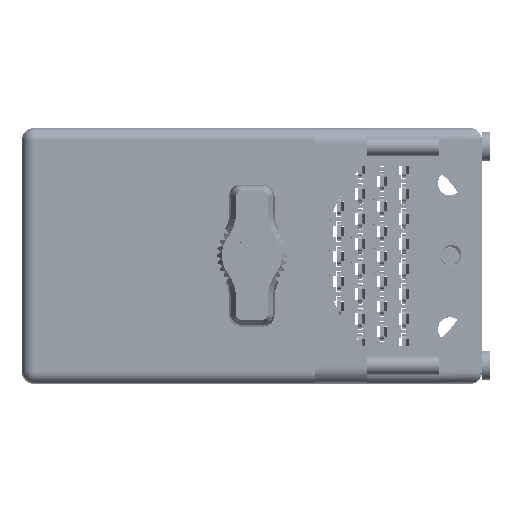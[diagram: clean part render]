
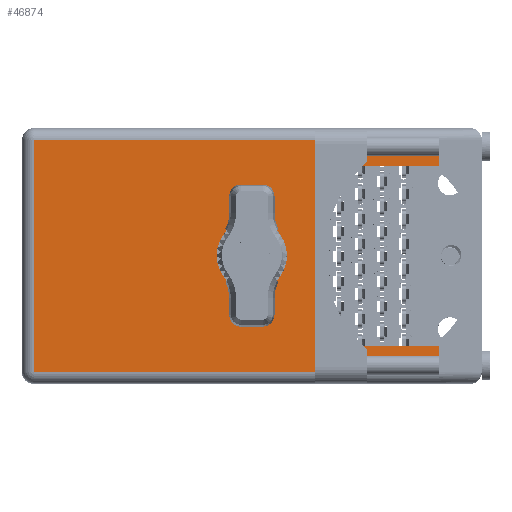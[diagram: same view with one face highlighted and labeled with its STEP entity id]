
A CAD part, top view. The second image highlights one B-rep face of the part: STEP entity #46874.
In plain terms, the highlighted face is planar.
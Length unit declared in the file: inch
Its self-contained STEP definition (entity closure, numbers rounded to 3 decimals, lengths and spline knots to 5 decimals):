
#1125 = AXIS2_PLACEMENT_3D ( 'NONE', #104734, #112836, #76635 ) ;
#4135 = VECTOR ( 'NONE', #70234, 39.37008 ) ;
#5523 = LINE ( 'NONE', #11830, #114775 ) ;
#6283 = VERTEX_POINT ( 'NONE', #26137 ) ;
#6298 = ORIENTED_EDGE ( 'NONE', *, *, #83334, .T. ) ;
#6409 = CARTESIAN_POINT ( 'NONE',  ( 0., 2.03, -1.46 ) ) ;
#7267 = EDGE_LOOP ( 'NONE', ( #102553, #46336, #51465, #106313, #6298, #98433, #116353, #37345 ) ) ;
#8203 = FACE_OUTER_BOUND ( 'NONE', #7267, .T. ) ;
#11830 = CARTESIAN_POINT ( 'NONE',  ( 2.499, 2.03, -1.53 ) ) ;
#12040 = VERTEX_POINT ( 'NONE', #65468 ) ;
#12286 = DIRECTION ( 'NONE',  ( 0., 0., 1. ) ) ;
#13913 = DIRECTION ( 'NONE',  ( 1., 0., 0. ) ) ;
#14869 = AXIS2_PLACEMENT_3D ( 'NONE', #26326, #91698, #35179 ) ;
#18072 = EDGE_CURVE ( 'NONE', #61223, #6283, #25681, .T. ) ;
#21875 = LINE ( 'NONE', #77321, #57810 ) ;
#22749 = CARTESIAN_POINT ( 'NONE',  ( 1.785, 2.03, -1.305 ) ) ;
#23350 = CARTESIAN_POINT ( 'NONE',  ( 2.499, 2.03, -0.07 ) ) ;
#23703 = EDGE_CURVE ( 'NONE', #98902, #97564, #72980, .T. ) ;
#24922 = CARTESIAN_POINT ( 'NONE',  ( 2.499, 2.03, -0.225 ) ) ;
#25681 = LINE ( 'NONE', #108618, #110474 ) ;
#26137 = CARTESIAN_POINT ( 'NONE',  ( 0.07, 2.03, -0.07 ) ) ;
#26326 = CARTESIAN_POINT ( 'NONE',  ( 1.3775, 2.03, -0.765 ) ) ;
#28358 = ORIENTED_EDGE ( 'NONE', *, *, #86660, .F. ) ;
#30281 = CARTESIAN_POINT ( 'NONE',  ( 0., 2.03, -1.53 ) ) ;
#33749 = VERTEX_POINT ( 'NONE', #23350 ) ;
#34765 = EDGE_CURVE ( 'NONE', #115130, #12040, #5523, .T. ) ;
#35179 = DIRECTION ( 'NONE',  ( 0., 0., 1. ) ) ;
#35689 = LINE ( 'NONE', #69709, #47110 ) ;
#36086 = CARTESIAN_POINT ( 'NONE',  ( 1.3775, 2.03, -0.595 ) ) ;
#37345 = ORIENTED_EDGE ( 'NONE', *, *, #74358, .T. ) ;
#39644 = LINE ( 'NONE', #112432, #76914 ) ;
#39777 = VERTEX_POINT ( 'NONE', #24922 ) ;
#40352 = EDGE_CURVE ( 'NONE', #39777, #45033, #72244, .T. ) ;
#44731 = VERTEX_POINT ( 'NONE', #115864 ) ;
#45033 = VERTEX_POINT ( 'NONE', #94032 ) ;
#45855 = CIRCLE ( 'NONE', #1125, 0.17 ) ;
#46336 = ORIENTED_EDGE ( 'NONE', *, *, #48049, .T. ) ;
#46874 = ADVANCED_FACE ( 'NONE', ( #8203, #78607 ), #112604, .T. ) ;
#47110 = VECTOR ( 'NONE', #13913, 39.37008 ) ;
#48049 = EDGE_CURVE ( 'NONE', #6283, #33749, #39644, .T. ) ;
#49208 = VECTOR ( 'NONE', #86919, 39.37008 ) ;
#51465 = ORIENTED_EDGE ( 'NONE', *, *, #97383, .F. ) ;
#52544 = CARTESIAN_POINT ( 'NONE',  ( 0.07, 2.03, -1.46 ) ) ;
#53623 = VECTOR ( 'NONE', #109043, 39.37008 ) ;
#57429 = DIRECTION ( 'NONE',  ( 1., 0., 0. ) ) ;
#57810 = VECTOR ( 'NONE', #12286, 39.37008 ) ;
#61223 = VERTEX_POINT ( 'NONE', #52544 ) ;
#65468 = CARTESIAN_POINT ( 'NONE',  ( 2.499, 2.03, -1.305 ) ) ;
#65656 = DIRECTION ( 'NONE',  ( 0., 0., 1. ) ) ;
#69709 = CARTESIAN_POINT ( 'NONE',  ( 2.499, 2.03, -1.305 ) ) ;
#70234 = DIRECTION ( 'NONE',  ( -1., 0., 0. ) ) ;
#72244 = LINE ( 'NONE', #107843, #53623 ) ;
#72980 = CIRCLE ( 'NONE', #14869, 0.17 ) ;
#74358 = EDGE_CURVE ( 'NONE', #115130, #61223, #111857, .T. ) ;
#74712 = EDGE_CURVE ( 'NONE', #44731, #12040, #35689, .T. ) ;
#76635 = DIRECTION ( 'NONE',  ( 0., 0., 1. ) ) ;
#76914 = VECTOR ( 'NONE', #57429, 39.37008 ) ;
#77321 = CARTESIAN_POINT ( 'NONE',  ( 2.499, 2.03, -1.53 ) ) ;
#78607 = FACE_BOUND ( 'NONE', #107904, .T. ) ;
#78667 = CARTESIAN_POINT ( 'NONE',  ( 2.499, 2.03, -1.46 ) ) ;
#83334 = EDGE_CURVE ( 'NONE', #45033, #44731, #106625, .T. ) ;
#84444 = DIRECTION ( 'NONE',  ( 0., 0., 1. ) ) ;
#86660 = EDGE_CURVE ( 'NONE', #97564, #98902, #45855, .T. ) ;
#86919 = DIRECTION ( 'NONE',  ( 0., 0., -1. ) ) ;
#91698 = DIRECTION ( 'NONE',  ( 0., 1., 0. ) ) ;
#94032 = CARTESIAN_POINT ( 'NONE',  ( 1.785, 2.03, -0.225 ) ) ;
#95236 = DIRECTION ( 'NONE',  ( 0., 1., 0. ) ) ;
#96537 = CARTESIAN_POINT ( 'NONE',  ( 1.3775, 2.03, -0.935 ) ) ;
#97383 = EDGE_CURVE ( 'NONE', #39777, #33749, #21875, .T. ) ;
#97564 = VERTEX_POINT ( 'NONE', #96537 ) ;
#98433 = ORIENTED_EDGE ( 'NONE', *, *, #74712, .T. ) ;
#98902 = VERTEX_POINT ( 'NONE', #36086 ) ;
#99405 = AXIS2_PLACEMENT_3D ( 'NONE', #30281, #95236, #84444 ) ;
#102553 = ORIENTED_EDGE ( 'NONE', *, *, #18072, .T. ) ;
#104734 = CARTESIAN_POINT ( 'NONE',  ( 1.3775, 2.03, -0.765 ) ) ;
#105024 = ORIENTED_EDGE ( 'NONE', *, *, #23703, .F. ) ;
#106313 = ORIENTED_EDGE ( 'NONE', *, *, #40352, .T. ) ;
#106625 = LINE ( 'NONE', #22749, #49208 ) ;
#107843 = CARTESIAN_POINT ( 'NONE',  ( 2.499, 2.03, -0.225 ) ) ;
#107904 = EDGE_LOOP ( 'NONE', ( #105024, #28358 ) ) ;
#108219 = DIRECTION ( 'NONE',  ( 0., 0., 1. ) ) ;
#108618 = CARTESIAN_POINT ( 'NONE',  ( 0.07, 2.03, -1.53 ) ) ;
#109043 = DIRECTION ( 'NONE',  ( -1., 0., 0. ) ) ;
#110474 = VECTOR ( 'NONE', #108219, 39.37008 ) ;
#111857 = LINE ( 'NONE', #6409, #4135 ) ;
#112432 = CARTESIAN_POINT ( 'NONE',  ( 2.499, 2.03, -0.07 ) ) ;
#112604 = PLANE ( 'NONE',  #99405 ) ;
#112836 = DIRECTION ( 'NONE',  ( 0., 1., 0. ) ) ;
#114775 = VECTOR ( 'NONE', #65656, 39.37008 ) ;
#115130 = VERTEX_POINT ( 'NONE', #78667 ) ;
#115864 = CARTESIAN_POINT ( 'NONE',  ( 1.785, 2.03, -1.305 ) ) ;
#116353 = ORIENTED_EDGE ( 'NONE', *, *, #34765, .F. ) ;
